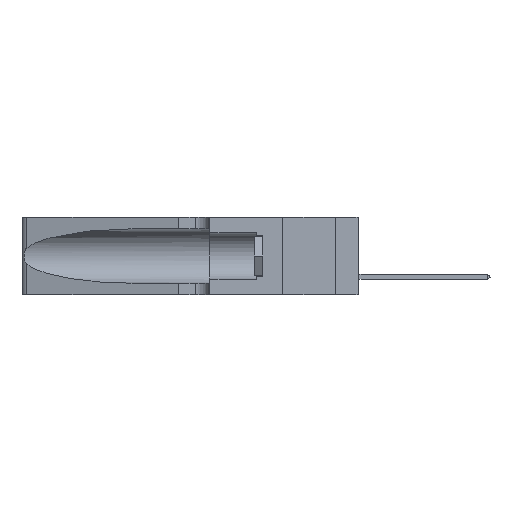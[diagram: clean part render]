
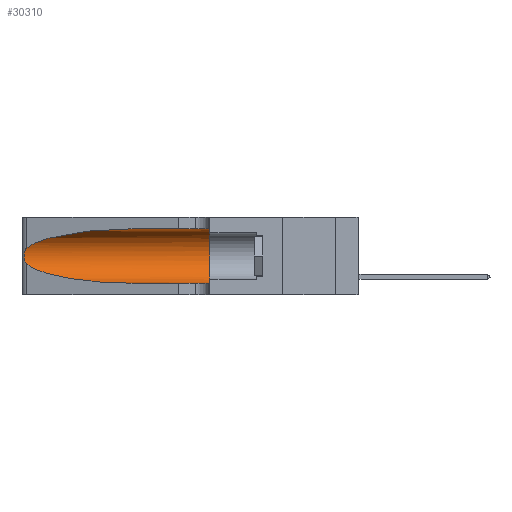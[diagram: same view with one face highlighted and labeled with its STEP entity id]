
A CAD part, left-side view. The second image highlights one B-rep face of the part: STEP entity #30310.
In plain terms, the highlighted cylindrical face has radius 3.308 mm (diameter 6.617 mm), a partial arc.
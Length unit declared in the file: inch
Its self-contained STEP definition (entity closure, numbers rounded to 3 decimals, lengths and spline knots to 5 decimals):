
#150 = AXIS2_PLACEMENT_3D ( 'NONE', #24388, #22050, #24890 ) ;
#216 = ORIENTED_EDGE ( 'NONE', *, *, #29599, .T. ) ;
#568 = CARTESIAN_POINT ( 'NONE',  ( 0.25487, 1.22718, 0.14631 ) ) ;
#1254 = CARTESIAN_POINT ( 'NONE',  ( 0.2373, 1.15595, 0.08982 ) ) ;
#1269 = EDGE_CURVE ( 'NONE', #31693, #20055, #11104, .T. ) ;
#1664 = VERTEX_POINT ( 'NONE', #568 ) ;
#2185 = EDGE_LOOP ( 'NONE', ( #15209, #216, #8857, #33991, #17256, #19014 ) ) ;
#4592 = AXIS2_PLACEMENT_3D ( 'NONE', #16203, #24671, #30062 ) ;
#4666 = CARTESIAN_POINT ( 'NONE',  ( 0.25555, 1.22994, 0.2215 ) ) ;
#5912 = CARTESIAN_POINT ( 'NONE',  ( 0.25487, 1.22718, 0.22369 ) ) ;
#7022 = EDGE_CURVE ( 'NONE', #27515, #20055, #11424, .T. ) ;
#7325 = CARTESIAN_POINT ( 'NONE',  ( 0.1305, 0.35, 0.05475 ) ) ;
#7596 = DIRECTION ( 'NONE',  ( 0., -1., 0. ) ) ;
#7641 = CARTESIAN_POINT ( 'NONE',  ( 0.25555, 1.22993, 0.14849 ) ) ;
#8857 = ORIENTED_EDGE ( 'NONE', *, *, #13091, .T. ) ;
#9840 = DIRECTION ( 'NONE',  ( 0., -1., 0. ) ) ;
#11104 = LINE ( 'NONE', #21338, #21196 ) ;
#11424 = CIRCLE ( 'NONE', #150, 0.13025 ) ;
#12813 = CARTESIAN_POINT ( 'NONE',  ( 0.18966, 0.96281, 0.05475 ) ) ;
#13091 = EDGE_CURVE ( 'NONE', #1664, #31693, #24441, .T. ) ;
#13119 = CARTESIAN_POINT ( 'NONE',  ( 0.18966, 0.96281, 0.31525 ) ) ;
#15209 = ORIENTED_EDGE ( 'NONE', *, *, #17027, .T. ) ;
#16123 = CARTESIAN_POINT ( 'NONE',  ( 0.25854, 1.2359, 0.20912 ) ) ;
#16203 = CARTESIAN_POINT ( 'NONE',  ( 0.1305, 1.61858, 0.185 ) ) ;
#16279 = CARTESIAN_POINT ( 'NONE',  ( 0.1305, 0.35, 0.31525 ) ) ;
#17027 = EDGE_CURVE ( 'NONE', #31356, #26194, #17418, .T. ) ;
#17256 = ORIENTED_EDGE ( 'NONE', *, *, #7022, .F. ) ;
#17418 =( BOUNDED_CURVE ( )  B_SPLINE_CURVE ( 3, ( #21708, #13119, #30190, #33273 ),
 .UNSPECIFIED., .F., .T. ) 
 B_SPLINE_CURVE_WITH_KNOTS ( ( 4, 4 ),
 ( 1.5708, 2.84003 ),
 .UNSPECIFIED. ) 
 CURVE ( )  GEOMETRIC_REPRESENTATION_ITEM ( )  RATIONAL_B_SPLINE_CURVE ( ( 1., 0.87, 0.87, 1. ) ) 
 REPRESENTATION_ITEM ( '' )  );
#18163 = CARTESIAN_POINT ( 'NONE',  ( 0.1305, 0.72297, 0.31525 ) ) ;
#18837 = CARTESIAN_POINT ( 'NONE',  ( 0.25789, 1.23486, 0.15765 ) ) ;
#19014 = ORIENTED_EDGE ( 'NONE', *, *, #33409, .F. ) ;
#19195 = CARTESIAN_POINT ( 'NONE',  ( 0.26075, 1.23896, 0.178 ) ) ;
#20055 = VERTEX_POINT ( 'NONE', #7325 ) ;
#21196 = VECTOR ( 'NONE', #9840, 39.37008 ) ;
#21330 = CARTESIAN_POINT ( 'NONE',  ( 0.1305, 1.61858, 0.31525 ) ) ;
#21338 = CARTESIAN_POINT ( 'NONE',  ( 0.1305, 1.61858, 0.05475 ) ) ;
#21708 = CARTESIAN_POINT ( 'NONE',  ( 0.1305, 0.72297, 0.31525 ) ) ;
#21747 = CARTESIAN_POINT ( 'NONE',  ( 0.25856, 1.23593, 0.16098 ) ) ;
#22001 = CARTESIAN_POINT ( 'NONE',  ( 0.25787, 1.23484, 0.2124 ) ) ;
#22050 = DIRECTION ( 'NONE',  ( 0., 1., 0. ) ) ;
#24388 = CARTESIAN_POINT ( 'NONE',  ( 0.1305, 0.35, 0.185 ) ) ;
#24441 =( BOUNDED_CURVE ( )  B_SPLINE_CURVE ( 3, ( #26828, #1254, #12813, #35421 ),
 .UNSPECIFIED., .F., .T. ) 
 B_SPLINE_CURVE_WITH_KNOTS ( ( 4, 4 ),
 ( 3.44316, 4.71239 ),
 .UNSPECIFIED. ) 
 CURVE ( )  GEOMETRIC_REPRESENTATION_ITEM ( )  RATIONAL_B_SPLINE_CURVE ( ( 1., 0.87, 0.87, 1. ) ) 
 REPRESENTATION_ITEM ( '' )  );
#24671 = DIRECTION ( 'NONE',  ( 0., -1., 0. ) ) ;
#24839 = CARTESIAN_POINT ( 'NONE',  ( 0.26017, 1.23833, 0.17102 ) ) ;
#24890 = DIRECTION ( 'NONE',  ( 0., 0., 1. ) ) ;
#26194 = VERTEX_POINT ( 'NONE', #5912 ) ;
#26828 = CARTESIAN_POINT ( 'NONE',  ( 0.25487, 1.22718, 0.14631 ) ) ;
#27271 = CARTESIAN_POINT ( 'NONE',  ( 0.25487, 1.22718, 0.22369 ) ) ;
#27515 = VERTEX_POINT ( 'NONE', #16279 ) ;
#27644 = CARTESIAN_POINT ( 'NONE',  ( 0.26018, 1.23835, 0.19895 ) ) ;
#27760 = FACE_OUTER_BOUND ( 'NONE', #2185, .T. ) ;
#28774 = VECTOR ( 'NONE', #7596, 39.37008 ) ;
#29599 = EDGE_CURVE ( 'NONE', #26194, #1664, #35448, .T. ) ;
#29982 = CARTESIAN_POINT ( 'NONE',  ( 0.25639, 1.23186, 0.15144 ) ) ;
#30062 = DIRECTION ( 'NONE',  ( 0., 0., -1. ) ) ;
#30190 = CARTESIAN_POINT ( 'NONE',  ( 0.2373, 1.15595, 0.28018 ) ) ;
#30238 = CARTESIAN_POINT ( 'NONE',  ( 0.25639, 1.23184, 0.21858 ) ) ;
#30310 = ADVANCED_FACE ( 'NONE', ( #27760 ), #36124, .F. ) ;
#30357 = CARTESIAN_POINT ( 'NONE',  ( 0.26075, 1.23896, 0.19203 ) ) ;
#30991 = CARTESIAN_POINT ( 'NONE',  ( 0.1305, 0.72297, 0.05475 ) ) ;
#31356 = VERTEX_POINT ( 'NONE', #18163 ) ;
#31693 = VERTEX_POINT ( 'NONE', #30991 ) ;
#32803 = CARTESIAN_POINT ( 'NONE',  ( 0.25487, 1.22718, 0.14631 ) ) ;
#33273 = CARTESIAN_POINT ( 'NONE',  ( 0.25487, 1.22718, 0.22369 ) ) ;
#33409 = EDGE_CURVE ( 'NONE', #31356, #27515, #35425, .T. ) ;
#33991 = ORIENTED_EDGE ( 'NONE', *, *, #1269, .T. ) ;
#35421 = CARTESIAN_POINT ( 'NONE',  ( 0.1305, 0.72297, 0.05475 ) ) ;
#35425 = LINE ( 'NONE', #21330, #28774 ) ;
#35448 = B_SPLINE_CURVE_WITH_KNOTS ( 'NONE', 3,
 ( #27271, #4666, #30238, #22001, #16123, #27644, #30357, #19195, #24839, #21747, #18837, #29982, #7641, #32803 ),
 .UNSPECIFIED., .F., .F.,
 ( 4, 2, 2, 2, 2, 2, 4 ),
 ( 0., 0.00027, 0.00053, 0.00107, 0.0016, 0.00187, 0.00214 ),
 .UNSPECIFIED. ) ;
#36124 = CYLINDRICAL_SURFACE ( 'NONE', #4592, 0.13025 ) ;
